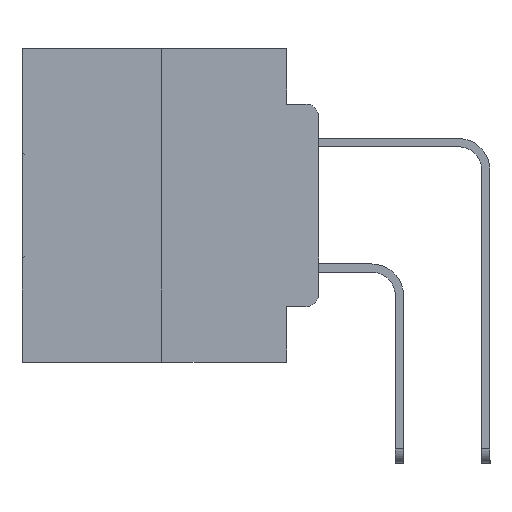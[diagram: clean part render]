
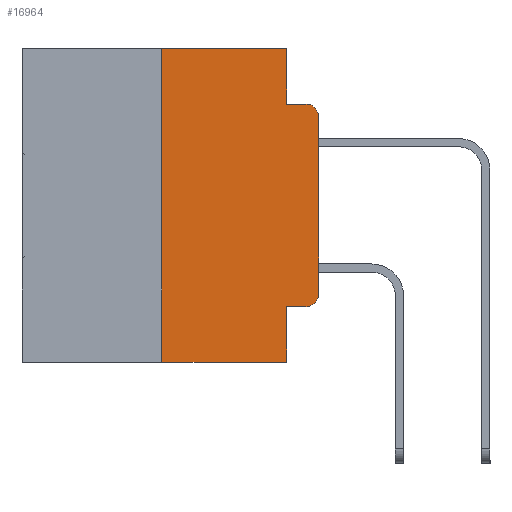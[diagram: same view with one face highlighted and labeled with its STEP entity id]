
A CAD part, left-side view. The second image highlights one B-rep face of the part: STEP entity #16964.
In plain terms, the highlighted planar face has unit normal (-1, 0, 0).
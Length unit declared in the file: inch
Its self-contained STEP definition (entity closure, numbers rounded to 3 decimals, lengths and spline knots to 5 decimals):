
#27 = VECTOR ( 'NONE', #4940, 39.37008 ) ;
#202 = ORIENTED_EDGE ( 'NONE', *, *, #19099, .T. ) ;
#1854 = ORIENTED_EDGE ( 'NONE', *, *, #30553, .T. ) ;
#2164 = DIRECTION ( 'NONE',  ( -1., 0., 0. ) ) ;
#3160 = AXIS2_PLACEMENT_3D ( 'NONE', #16942, #4290, #21824 ) ;
#3505 = VECTOR ( 'NONE', #19906, 39.37008 ) ;
#3540 = LINE ( 'NONE', #7394, #10330 ) ;
#4290 = DIRECTION ( 'NONE',  ( 1., 0., 0. ) ) ;
#4940 = DIRECTION ( 'NONE',  ( 0., 0., 1. ) ) ;
#5203 = VECTOR ( 'NONE', #15949, 39.37008 ) ;
#5433 = ORIENTED_EDGE ( 'NONE', *, *, #24313, .F. ) ;
#5524 = VERTEX_POINT ( 'NONE', #8926 ) ;
#5805 = VERTEX_POINT ( 'NONE', #12609 ) ;
#5928 = VERTEX_POINT ( 'NONE', #22851 ) ;
#6142 = VERTEX_POINT ( 'NONE', #11376 ) ;
#6520 = VERTEX_POINT ( 'NONE', #23046 ) ;
#6678 = LINE ( 'NONE', #25282, #20095 ) ;
#6849 = VERTEX_POINT ( 'NONE', #14525 ) ;
#6860 = LINE ( 'NONE', #27139, #27 ) ;
#7394 = CARTESIAN_POINT ( 'NONE',  ( 0., 0.473, -0.5 ) ) ;
#7421 = ORIENTED_EDGE ( 'NONE', *, *, #9379, .T. ) ;
#8798 = CIRCLE ( 'NONE', #17121, 0.02 ) ;
#8926 = CARTESIAN_POINT ( 'NONE',  ( 0., 0.051, 0. ) ) ;
#9379 = EDGE_CURVE ( 'NONE', #6849, #5928, #6860, .T. ) ;
#10291 = LINE ( 'NONE', #26999, #3505 ) ;
#10330 = VECTOR ( 'NONE', #24785, 39.37008 ) ;
#10510 = DIRECTION ( 'NONE',  ( 0., -1., 0. ) ) ;
#10940 = VERTEX_POINT ( 'NONE', #12006 ) ;
#11376 = CARTESIAN_POINT ( 'NONE',  ( 0., 0.25, -0.5 ) ) ;
#11752 = DIRECTION ( 'NONE',  ( 0., -1., 0. ) ) ;
#12006 = CARTESIAN_POINT ( 'NONE',  ( 0., 0.02, -0.0885 ) ) ;
#12228 = DIRECTION ( 'NONE',  ( -1., 0., 0. ) ) ;
#12609 = CARTESIAN_POINT ( 'NONE',  ( 0., 0.051, -0.5 ) ) ;
#12818 = EDGE_CURVE ( 'NONE', #5928, #10940, #8798, .T. ) ;
#13809 = CARTESIAN_POINT ( 'NONE',  ( 0., 0.02, -0.4115 ) ) ;
#13824 = ORIENTED_EDGE ( 'NONE', *, *, #25939, .F. ) ;
#14483 = EDGE_CURVE ( 'NONE', #22836, #10940, #6678, .T. ) ;
#14525 = CARTESIAN_POINT ( 'NONE',  ( 0., 0., -0.3915 ) ) ;
#14912 = EDGE_LOOP ( 'NONE', ( #7421, #14985, #29259, #24553, #5433, #19668, #202, #13824, #27484, #1854 ) ) ;
#14985 = ORIENTED_EDGE ( 'NONE', *, *, #12818, .T. ) ;
#15949 = DIRECTION ( 'NONE',  ( 0., -1., 0. ) ) ;
#16942 = CARTESIAN_POINT ( 'NONE',  ( 0., 0.473, 0. ) ) ;
#16964 = ADVANCED_FACE ( 'NONE', ( #19981 ), #28853, .F. ) ;
#17121 = AXIS2_PLACEMENT_3D ( 'NONE', #17378, #2164, #19859 ) ;
#17378 = CARTESIAN_POINT ( 'NONE',  ( 0., 0.02, -0.1085 ) ) ;
#17624 = CARTESIAN_POINT ( 'NONE',  ( 0., 0.25, 0. ) ) ;
#17660 = DIRECTION ( 'NONE',  ( 0., 0., -1. ) ) ;
#17860 = VECTOR ( 'NONE', #17660, 39.37008 ) ;
#17867 = EDGE_CURVE ( 'NONE', #5524, #22836, #24301, .T. ) ;
#18744 = LINE ( 'NONE', #21701, #24397 ) ;
#18748 = AXIS2_PLACEMENT_3D ( 'NONE', #26865, #12228, #29149 ) ;
#19099 = EDGE_CURVE ( 'NONE', #6142, #5805, #3540, .T. ) ;
#19513 = EDGE_CURVE ( 'NONE', #6142, #29642, #10291, .T. ) ;
#19668 = ORIENTED_EDGE ( 'NONE', *, *, #19513, .F. ) ;
#19859 = DIRECTION ( 'NONE',  ( 0., 0., -1. ) ) ;
#19906 = DIRECTION ( 'NONE',  ( 0., 0., 1. ) ) ;
#19981 = FACE_OUTER_BOUND ( 'NONE', #14912, .T. ) ;
#20095 = VECTOR ( 'NONE', #10510, 39.37008 ) ;
#20512 = VECTOR ( 'NONE', #29882, 39.37008 ) ;
#21701 = CARTESIAN_POINT ( 'NONE',  ( 0., 0.051, -0.4115 ) ) ;
#21824 = DIRECTION ( 'NONE',  ( 0., 0., -1. ) ) ;
#22123 = CARTESIAN_POINT ( 'NONE',  ( 0., 0.051, -0.0885 ) ) ;
#22734 = EDGE_CURVE ( 'NONE', #6520, #29323, #18744, .T. ) ;
#22836 = VERTEX_POINT ( 'NONE', #22123 ) ;
#22851 = CARTESIAN_POINT ( 'NONE',  ( 0., 0., -0.1085 ) ) ;
#23046 = CARTESIAN_POINT ( 'NONE',  ( 0., 0.051, -0.4115 ) ) ;
#24301 = LINE ( 'NONE', #24967, #17860 ) ;
#24313 = EDGE_CURVE ( 'NONE', #29642, #5524, #29776, .T. ) ;
#24397 = VECTOR ( 'NONE', #11752, 39.37008 ) ;
#24553 = ORIENTED_EDGE ( 'NONE', *, *, #17867, .F. ) ;
#24785 = DIRECTION ( 'NONE',  ( 0., -1., 0. ) ) ;
#24967 = CARTESIAN_POINT ( 'NONE',  ( 0., 0.051, 0. ) ) ;
#25282 = CARTESIAN_POINT ( 'NONE',  ( 0., 0.051, -0.0885 ) ) ;
#25939 = EDGE_CURVE ( 'NONE', #6520, #5805, #26861, .T. ) ;
#26861 = LINE ( 'NONE', #27590, #20512 ) ;
#26865 = CARTESIAN_POINT ( 'NONE',  ( 0., 0.02, -0.3915 ) ) ;
#26999 = CARTESIAN_POINT ( 'NONE',  ( 0., 0.25, 0. ) ) ;
#27139 = CARTESIAN_POINT ( 'NONE',  ( 0., 0., 0. ) ) ;
#27484 = ORIENTED_EDGE ( 'NONE', *, *, #22734, .T. ) ;
#27590 = CARTESIAN_POINT ( 'NONE',  ( 0., 0.051, 0. ) ) ;
#28853 = PLANE ( 'NONE',  #3160 ) ;
#29149 = DIRECTION ( 'NONE',  ( 0., 0., -1. ) ) ;
#29259 = ORIENTED_EDGE ( 'NONE', *, *, #14483, .F. ) ;
#29323 = VERTEX_POINT ( 'NONE', #13809 ) ;
#29642 = VERTEX_POINT ( 'NONE', #17624 ) ;
#29776 = LINE ( 'NONE', #30245, #5203 ) ;
#29882 = DIRECTION ( 'NONE',  ( 0., 0., -1. ) ) ;
#30245 = CARTESIAN_POINT ( 'NONE',  ( 0., 0.473, 0. ) ) ;
#30425 = CIRCLE ( 'NONE', #18748, 0.02 ) ;
#30553 = EDGE_CURVE ( 'NONE', #29323, #6849, #30425, .T. ) ;
